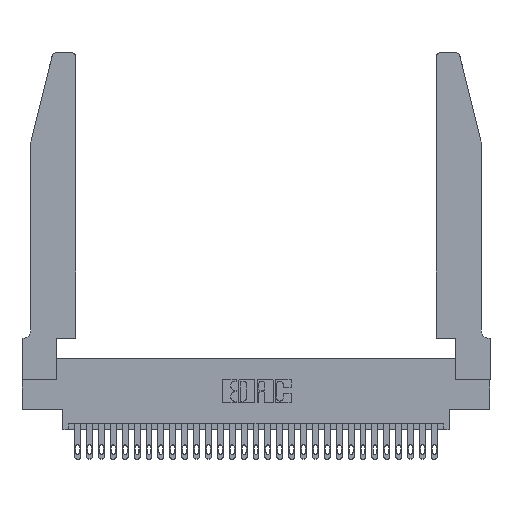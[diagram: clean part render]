
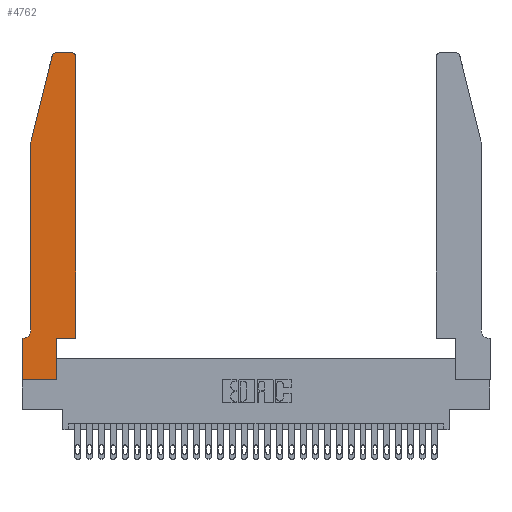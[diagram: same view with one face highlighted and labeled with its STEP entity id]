
A CAD part, top view. The second image highlights one B-rep face of the part: STEP entity #4762.
In plain terms, the highlighted planar face has unit normal (0, 0, 1).
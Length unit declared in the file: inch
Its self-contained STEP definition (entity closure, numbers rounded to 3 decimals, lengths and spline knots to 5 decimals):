
#263 = VERTEX_POINT ( 'NONE', #28170 ) ;
#471 = DIRECTION ( 'NONE',  ( -1., 0., 0. ) ) ;
#549 = CIRCLE ( 'NONE', #24393, 0.07 ) ;
#615 = EDGE_CURVE ( 'NONE', #263, #22985, #3854, .T. ) ;
#996 = AXIS2_PLACEMENT_3D ( 'NONE', #12852, #15236, #17615 ) ;
#1070 = EDGE_LOOP ( 'NONE', ( #22826, #10299, #7623, #7115, #16806, #25384, #6938, #3273, #15202, #18979, #27093, #11112 ) ) ;
#1261 = VECTOR ( 'NONE', #4602, 39.37008 ) ;
#1279 = CARTESIAN_POINT ( 'NONE',  ( 0.0755, 0.42, 0.37 ) ) ;
#2076 = LINE ( 'NONE', #10944, #13162 ) ;
#2285 = CARTESIAN_POINT ( 'NONE',  ( 0.284, 2.75, 0.37 ) ) ;
#2533 = VERTEX_POINT ( 'NONE', #2285 ) ;
#2706 = CARTESIAN_POINT ( 'NONE',  ( 0.4505, 2.72, 0.37 ) ) ;
#2764 = LINE ( 'NONE', #12576, #17593 ) ;
#2926 = CIRCLE ( 'NONE', #6874, 0.03 ) ;
#3273 = ORIENTED_EDGE ( 'NONE', *, *, #21315, .T. ) ;
#3436 = DIRECTION ( 'NONE',  ( -0.239, -0.971, 0. ) ) ;
#3854 = LINE ( 'NONE', #20565, #28288 ) ;
#4410 = DIRECTION ( 'NONE',  ( 0., 1., 0. ) ) ;
#4602 = DIRECTION ( 'NONE',  ( 1., 0., 0. ) ) ;
#4762 = ADVANCED_FACE ( 'NONE', ( #4844 ), #8116, .T. ) ;
#4844 = FACE_OUTER_BOUND ( 'NONE', #1070, .T. ) ;
#5043 = EDGE_CURVE ( 'NONE', #5614, #263, #10741, .T. ) ;
#5614 = VERTEX_POINT ( 'NONE', #24802 ) ;
#5975 = DIRECTION ( 'NONE',  ( 0., 1., 0. ) ) ;
#6014 = EDGE_CURVE ( 'NONE', #21293, #24828, #21114, .T. ) ;
#6538 = AXIS2_PLACEMENT_3D ( 'NONE', #12473, #17440, #24275 ) ;
#6688 = CARTESIAN_POINT ( 'NONE',  ( 0.2865, 0.35, 0.37 ) ) ;
#6849 = DIRECTION ( 'NONE',  ( 1., 0., 0. ) ) ;
#6874 = AXIS2_PLACEMENT_3D ( 'NONE', #21229, #16552, #6849 ) ;
#6938 = ORIENTED_EDGE ( 'NONE', *, *, #6014, .T. ) ;
#7115 = ORIENTED_EDGE ( 'NONE', *, *, #29228, .T. ) ;
#7236 = LINE ( 'NONE', #14820, #7989 ) ;
#7623 = ORIENTED_EDGE ( 'NONE', *, *, #26075, .T. ) ;
#7989 = VECTOR ( 'NONE', #3436, 39.37008 ) ;
#8116 = PLANE ( 'NONE',  #996 ) ;
#8480 = DIRECTION ( 'NONE',  ( 1., 0., 0. ) ) ;
#8590 = CARTESIAN_POINT ( 'NONE',  ( 0.4505, 0.35, 0.37 ) ) ;
#8747 = EDGE_CURVE ( 'NONE', #19869, #2533, #2764, .T. ) ;
#8772 = VERTEX_POINT ( 'NONE', #12914 ) ;
#8877 = EDGE_CURVE ( 'NONE', #19806, #21757, #549, .T. ) ;
#9391 = LINE ( 'NONE', #25808, #1261 ) ;
#10299 = ORIENTED_EDGE ( 'NONE', *, *, #18934, .T. ) ;
#10741 = LINE ( 'NONE', #8590, #27788 ) ;
#10944 = CARTESIAN_POINT ( 'NONE',  ( 0.0755, 0.35, 0.37 ) ) ;
#11112 = ORIENTED_EDGE ( 'NONE', *, *, #14687, .T. ) ;
#12387 = CARTESIAN_POINT ( 'NONE',  ( 0.0755, 2., 0.37 ) ) ;
#12473 = CARTESIAN_POINT ( 'NONE',  ( 0.284, 2.72, 0.37 ) ) ;
#12576 = CARTESIAN_POINT ( 'NONE',  ( 0.2605, 2.75, 0.37 ) ) ;
#12852 = CARTESIAN_POINT ( 'NONE',  ( 0., 0.35, 0.37 ) ) ;
#12914 = CARTESIAN_POINT ( 'NONE',  ( 0.2865, 0., 0.37 ) ) ;
#13162 = VECTOR ( 'NONE', #20274, 39.37008 ) ;
#13228 = DIRECTION ( 'NONE',  ( 0., -1., 0. ) ) ;
#13682 = CARTESIAN_POINT ( 'NONE',  ( 0.4205, 2.75, 0.37 ) ) ;
#13694 = LINE ( 'NONE', #6688, #20747 ) ;
#14477 = LINE ( 'NONE', #22397, #30414 ) ;
#14641 = DIRECTION ( 'NONE',  ( 0., 0., -1. ) ) ;
#14687 = EDGE_CURVE ( 'NONE', #22985, #19869, #2926, .T. ) ;
#14820 = CARTESIAN_POINT ( 'NONE',  ( 0.0755, 2., 0.37 ) ) ;
#15202 = ORIENTED_EDGE ( 'NONE', *, *, #18019, .T. ) ;
#15236 = DIRECTION ( 'NONE',  ( 0., 0., 1. ) ) ;
#15495 = CARTESIAN_POINT ( 'NONE',  ( 0., 0., 0.37 ) ) ;
#16552 = DIRECTION ( 'NONE',  ( 0., 0., 1. ) ) ;
#16806 = ORIENTED_EDGE ( 'NONE', *, *, #8877, .T. ) ;
#17440 = DIRECTION ( 'NONE',  ( 0., 0., 1. ) ) ;
#17593 = VECTOR ( 'NONE', #21790, 39.37008 ) ;
#17615 = DIRECTION ( 'NONE',  ( 1., 0., 0. ) ) ;
#18019 = EDGE_CURVE ( 'NONE', #8772, #5614, #13694, .T. ) ;
#18574 = CARTESIAN_POINT ( 'NONE',  ( 0., 0.35, 0.37 ) ) ;
#18934 = EDGE_CURVE ( 'NONE', #2533, #20647, #26586, .T. ) ;
#18979 = ORIENTED_EDGE ( 'NONE', *, *, #5043, .T. ) ;
#19611 = CARTESIAN_POINT ( 'NONE',  ( 0.0055, 0.42, 0.37 ) ) ;
#19806 = VERTEX_POINT ( 'NONE', #1279 ) ;
#19869 = VERTEX_POINT ( 'NONE', #13682 ) ;
#20274 = DIRECTION ( 'NONE',  ( -1., 0., 0. ) ) ;
#20435 = EDGE_CURVE ( 'NONE', #21757, #21293, #2076, .T. ) ;
#20565 = CARTESIAN_POINT ( 'NONE',  ( 0.4505, 0.35, 0.37 ) ) ;
#20647 = VERTEX_POINT ( 'NONE', #23188 ) ;
#20747 = VECTOR ( 'NONE', #4410, 39.37008 ) ;
#21114 = LINE ( 'NONE', #15495, #24436 ) ;
#21229 = CARTESIAN_POINT ( 'NONE',  ( 0.4205, 2.72, 0.37 ) ) ;
#21293 = VERTEX_POINT ( 'NONE', #18574 ) ;
#21315 = EDGE_CURVE ( 'NONE', #24828, #8772, #9391, .T. ) ;
#21757 = VERTEX_POINT ( 'NONE', #23500 ) ;
#21790 = DIRECTION ( 'NONE',  ( -1., 0., 0. ) ) ;
#22161 = CARTESIAN_POINT ( 'NONE',  ( 0., 0., 0.37 ) ) ;
#22397 = CARTESIAN_POINT ( 'NONE',  ( 0.0755, 2., 0.37 ) ) ;
#22826 = ORIENTED_EDGE ( 'NONE', *, *, #8747, .T. ) ;
#22985 = VERTEX_POINT ( 'NONE', #2706 ) ;
#23188 = CARTESIAN_POINT ( 'NONE',  ( 0.25487, 2.72718, 0.37 ) ) ;
#23500 = CARTESIAN_POINT ( 'NONE',  ( 0.0055, 0.35, 0.37 ) ) ;
#24275 = DIRECTION ( 'NONE',  ( 1., 0., 0. ) ) ;
#24393 = AXIS2_PLACEMENT_3D ( 'NONE', #19611, #14641, #471 ) ;
#24436 = VECTOR ( 'NONE', #13228, 39.37008 ) ;
#24773 = DIRECTION ( 'NONE',  ( 0., -1., 0. ) ) ;
#24802 = CARTESIAN_POINT ( 'NONE',  ( 0.2865, 0.35, 0.37 ) ) ;
#24828 = VERTEX_POINT ( 'NONE', #22161 ) ;
#25384 = ORIENTED_EDGE ( 'NONE', *, *, #20435, .T. ) ;
#25808 = CARTESIAN_POINT ( 'NONE',  ( 0., 0., 0.37 ) ) ;
#26075 = EDGE_CURVE ( 'NONE', #20647, #27180, #7236, .T. ) ;
#26586 = CIRCLE ( 'NONE', #6538, 0.03 ) ;
#27093 = ORIENTED_EDGE ( 'NONE', *, *, #615, .T. ) ;
#27180 = VERTEX_POINT ( 'NONE', #12387 ) ;
#27788 = VECTOR ( 'NONE', #8480, 39.37008 ) ;
#28170 = CARTESIAN_POINT ( 'NONE',  ( 0.4505, 0.35, 0.37 ) ) ;
#28288 = VECTOR ( 'NONE', #5975, 39.37008 ) ;
#29228 = EDGE_CURVE ( 'NONE', #27180, #19806, #14477, .T. ) ;
#30414 = VECTOR ( 'NONE', #24773, 39.37008 ) ;
